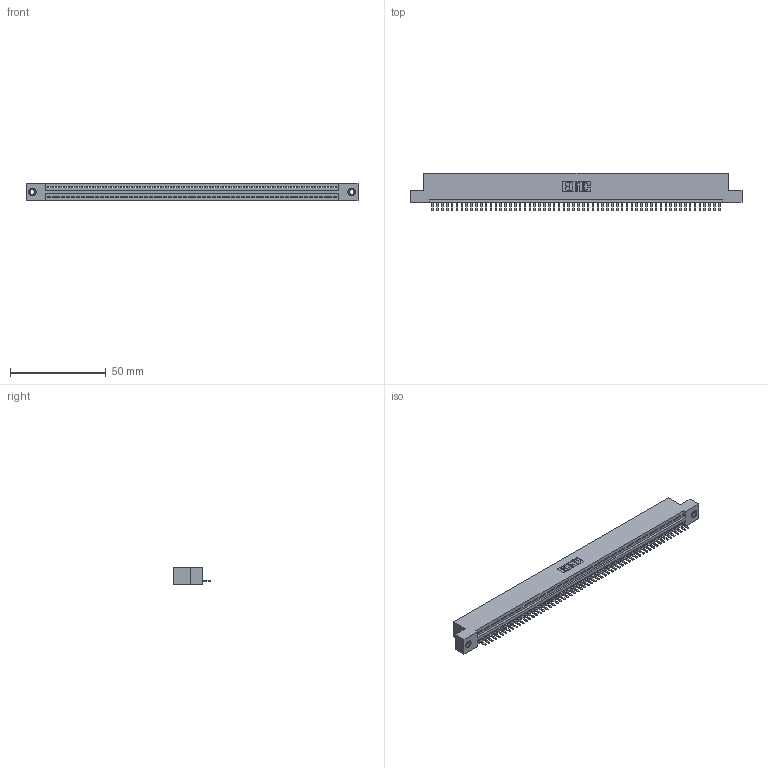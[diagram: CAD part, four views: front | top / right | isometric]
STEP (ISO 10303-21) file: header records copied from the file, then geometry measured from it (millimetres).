
FILE_DESCRIPTION (( 'STEP AP203' ), '1' );
FILE_NAME ('395-060-520-107.STEP', '2019-10-24T10:56:06', ( '' ), ( '' ), 'SwSTEP 2.0', 'SolidWorks 2016', '' );
FILE_SCHEMA (( 'CONFIG_CONTROL_DESIGN' ));
Length unit declared in the file: inch
Products named in the file (4): 395-060-520-107; 345-250-001_345-250-005-103; 345-292-001_345-293-120; 345 Part_Flush Mounting Lugs - 0.156 Dia-TI
Assembly tree (63 placements, depth 2):
  395-060-520-107
    345 Part_Flush Mounting Lugs - 0.156 Dia-TI
    345-292-001_345-293-120  x60
    345-250-001_345-250-005-103  x2
Bounding box: 173.61 x 19.68 x 9.4 mm (x, y, z)
Volume: 16450.9 mm3; surface area: 21574.3 mm2
Topology: 63 solids, 63 shells, 3906 faces, 11517 edges, 7510 vertices
Faces by surface type: plane 2632, cylinder 1258, cone 12, torus 4
Entity records: 44034 total; most frequent: CARTESIAN_POINT 7619, ORIENTED_EDGE 7594, DIRECTION 6643, EDGE_CURVE 3797, VECTOR 3401, LINE 3401, VERTEX_POINT 2524, AXIS2_PLACEMENT_3D 1621
